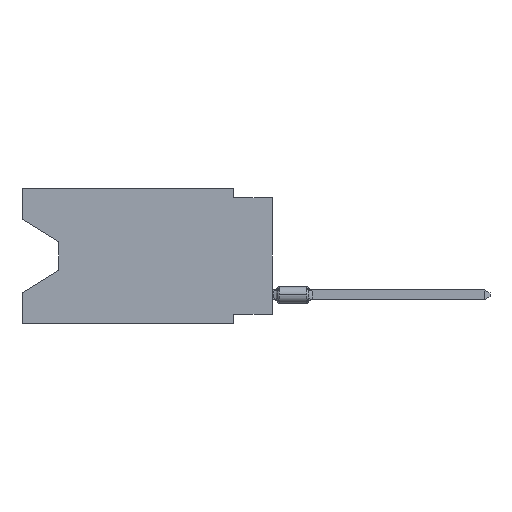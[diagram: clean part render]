
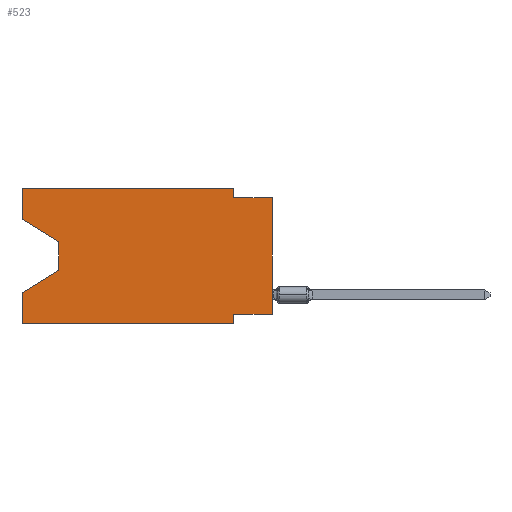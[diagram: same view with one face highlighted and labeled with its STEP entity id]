
A CAD part, left-side view. The second image highlights one B-rep face of the part: STEP entity #523.
In plain terms, the highlighted planar face has unit normal (-1, 0, 0).
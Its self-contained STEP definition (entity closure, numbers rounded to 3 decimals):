
#380 = CARTESIAN_POINT ( 'NONE',  ( 0., 0., 0. ) ) ;
#493 = LINE ( 'NONE', #771, #12851 ) ;
#523 = ADVANCED_FACE ( 'NONE', ( #7950 ), #8307, .F. ) ;
#771 = CARTESIAN_POINT ( 'NONE',  ( 0., 16.383, 0. ) ) ;
#862 = LINE ( 'NONE', #4709, #13440 ) ;
#910 = LINE ( 'NONE', #6839, #8087 ) ;
#1002 = DIRECTION ( 'NONE',  ( 0., 0., -1. ) ) ;
#1224 = VECTOR ( 'NONE', #12477, 1000. ) ;
#1636 = CARTESIAN_POINT ( 'NONE',  ( 0., 16.383, 0. ) ) ;
#1651 = LINE ( 'NONE', #12739, #6028 ) ;
#1801 = LINE ( 'NONE', #7372, #5210 ) ;
#2561 = DIRECTION ( 'NONE',  ( 0., 0., -1. ) ) ;
#2707 = VERTEX_POINT ( 'NONE', #6445 ) ;
#3018 = VERTEX_POINT ( 'NONE', #3959 ) ;
#3088 = EDGE_CURVE ( 'NONE', #11472, #11033, #13482, .T. ) ;
#3222 = LINE ( 'NONE', #380, #14191 ) ;
#3312 = CARTESIAN_POINT ( 'NONE',  ( 0., 2.54, -8.89 ) ) ;
#3368 = CARTESIAN_POINT ( 'NONE',  ( 0., 16.383, -8.89 ) ) ;
#3432 = VERTEX_POINT ( 'NONE', #9058 ) ;
#3959 = CARTESIAN_POINT ( 'NONE',  ( 0., 0., -0.635 ) ) ;
#4311 = VERTEX_POINT ( 'NONE', #3368 ) ;
#4621 = ORIENTED_EDGE ( 'NONE', *, *, #10980, .F. ) ;
#4701 = EDGE_CURVE ( 'NONE', #14227, #9244, #1801, .T. ) ;
#4709 = CARTESIAN_POINT ( 'NONE',  ( 0., 16.383, -8.89 ) ) ;
#5210 = VECTOR ( 'NONE', #7550, 1000. ) ;
#5760 = DIRECTION ( 'NONE',  ( 0., 0., 1. ) ) ;
#5878 = EDGE_CURVE ( 'NONE', #11033, #3018, #7645, .T. ) ;
#6028 = VECTOR ( 'NONE', #13936, 1000. ) ;
#6445 = CARTESIAN_POINT ( 'NONE',  ( 0., 16.383, -6.852 ) ) ;
#6839 = CARTESIAN_POINT ( 'NONE',  ( 0., 2.54, -8.89 ) ) ;
#6927 = CARTESIAN_POINT ( 'NONE',  ( 0., 16.383, 0. ) ) ;
#7225 = CARTESIAN_POINT ( 'NONE',  ( 0., 16.383, -2.038 ) ) ;
#7372 = CARTESIAN_POINT ( 'NONE',  ( 0., 0., -8.255 ) ) ;
#7377 = CARTESIAN_POINT ( 'NONE',  ( 0., 2.54, -8.255 ) ) ;
#7550 = DIRECTION ( 'NONE',  ( 0., 1., 0. ) ) ;
#7553 = CARTESIAN_POINT ( 'NONE',  ( 0., 0., -0.635 ) ) ;
#7578 = EDGE_CURVE ( 'NONE', #3432, #2707, #15790, .T. ) ;
#7645 = LINE ( 'NONE', #7553, #12222 ) ;
#7819 = ORIENTED_EDGE ( 'NONE', *, *, #7578, .T. ) ;
#7950 = FACE_OUTER_BOUND ( 'NONE', #14306, .T. ) ;
#8087 = VECTOR ( 'NONE', #1002, 1000. ) ;
#8307 = PLANE ( 'NONE',  #15240 ) ;
#9048 = EDGE_CURVE ( 'NONE', #10380, #13650, #10702, .T. ) ;
#9058 = CARTESIAN_POINT ( 'NONE',  ( 0., 13.97, -5.385 ) ) ;
#9244 = VERTEX_POINT ( 'NONE', #7377 ) ;
#9537 = DIRECTION ( 'NONE',  ( 0., 0., -1. ) ) ;
#9698 = LINE ( 'NONE', #1636, #17618 ) ;
#9793 = ORIENTED_EDGE ( 'NONE', *, *, #16725, .F. ) ;
#10380 = VERTEX_POINT ( 'NONE', #10999 ) ;
#10542 = CARTESIAN_POINT ( 'NONE',  ( 0., 2.54, 0. ) ) ;
#10702 = LINE ( 'NONE', #6927, #16980 ) ;
#10900 = EDGE_CURVE ( 'NONE', #4311, #11404, #862, .T. ) ;
#10902 = ORIENTED_EDGE ( 'NONE', *, *, #13490, .T. ) ;
#10980 = EDGE_CURVE ( 'NONE', #13650, #11472, #493, .T. ) ;
#10999 = CARTESIAN_POINT ( 'NONE',  ( 0., 16.383, -2.038 ) ) ;
#11033 = VERTEX_POINT ( 'NONE', #13409 ) ;
#11309 = ORIENTED_EDGE ( 'NONE', *, *, #16516, .T. ) ;
#11404 = VERTEX_POINT ( 'NONE', #3312 ) ;
#11472 = VERTEX_POINT ( 'NONE', #13666 ) ;
#11852 = DIRECTION ( 'NONE',  ( 0., 0.855, -0.519 ) ) ;
#11953 = EDGE_CURVE ( 'NONE', #14227, #3018, #3222, .T. ) ;
#12042 = DIRECTION ( 'NONE',  ( 0., -1., 0. ) ) ;
#12222 = VECTOR ( 'NONE', #15806, 1000. ) ;
#12301 = CARTESIAN_POINT ( 'NONE',  ( 0., 13.97, -3.505 ) ) ;
#12477 = DIRECTION ( 'NONE',  ( 0., -0.855, -0.519 ) ) ;
#12481 = ORIENTED_EDGE ( 'NONE', *, *, #4701, .F. ) ;
#12739 = CARTESIAN_POINT ( 'NONE',  ( 0., 13.97, -3.505 ) ) ;
#12851 = VECTOR ( 'NONE', #14517, 1000. ) ;
#13409 = CARTESIAN_POINT ( 'NONE',  ( 0., 2.54, -0.635 ) ) ;
#13440 = VECTOR ( 'NONE', #12042, 1000. ) ;
#13482 = LINE ( 'NONE', #10542, #17153 ) ;
#13490 = EDGE_CURVE ( 'NONE', #10380, #17949, #15486, .T. ) ;
#13551 = DIRECTION ( 'NONE',  ( 0., 0., 1. ) ) ;
#13553 = DIRECTION ( 'NONE',  ( 1., 0., 0. ) ) ;
#13650 = VERTEX_POINT ( 'NONE', #15755 ) ;
#13666 = CARTESIAN_POINT ( 'NONE',  ( 0., 2.54, 0. ) ) ;
#13739 = ORIENTED_EDGE ( 'NONE', *, *, #3088, .F. ) ;
#13910 = CARTESIAN_POINT ( 'NONE',  ( 0., 16.383, 0. ) ) ;
#13936 = DIRECTION ( 'NONE',  ( 0., 0., -1. ) ) ;
#14191 = VECTOR ( 'NONE', #17146, 1000. ) ;
#14227 = VERTEX_POINT ( 'NONE', #16184 ) ;
#14306 = EDGE_LOOP ( 'NONE', ( #10902, #11309, #7819, #18057, #16222, #9793, #12481, #14565, #15036, #13739, #4621, #15047 ) ) ;
#14517 = DIRECTION ( 'NONE',  ( 0., -1., 0. ) ) ;
#14565 = ORIENTED_EDGE ( 'NONE', *, *, #11953, .T. ) ;
#15036 = ORIENTED_EDGE ( 'NONE', *, *, #5878, .F. ) ;
#15047 = ORIENTED_EDGE ( 'NONE', *, *, #9048, .F. ) ;
#15173 = EDGE_CURVE ( 'NONE', #4311, #2707, #9698, .T. ) ;
#15240 = AXIS2_PLACEMENT_3D ( 'NONE', #13910, #13553, #2561 ) ;
#15486 = LINE ( 'NONE', #7225, #1224 ) ;
#15755 = CARTESIAN_POINT ( 'NONE',  ( 0., 16.383, 0. ) ) ;
#15790 = LINE ( 'NONE', #17352, #17309 ) ;
#15806 = DIRECTION ( 'NONE',  ( 0., -1., 0. ) ) ;
#16184 = CARTESIAN_POINT ( 'NONE',  ( 0., 0., -8.255 ) ) ;
#16222 = ORIENTED_EDGE ( 'NONE', *, *, #10900, .T. ) ;
#16516 = EDGE_CURVE ( 'NONE', #17949, #3432, #1651, .T. ) ;
#16725 = EDGE_CURVE ( 'NONE', #9244, #11404, #910, .T. ) ;
#16980 = VECTOR ( 'NONE', #13551, 1000. ) ;
#17146 = DIRECTION ( 'NONE',  ( 0., 0., 1. ) ) ;
#17153 = VECTOR ( 'NONE', #9537, 1000. ) ;
#17309 = VECTOR ( 'NONE', #11852, 1000. ) ;
#17352 = CARTESIAN_POINT ( 'NONE',  ( 0., 13.97, -5.385 ) ) ;
#17618 = VECTOR ( 'NONE', #5760, 1000. ) ;
#17949 = VERTEX_POINT ( 'NONE', #12301 ) ;
#18057 = ORIENTED_EDGE ( 'NONE', *, *, #15173, .F. ) ;
